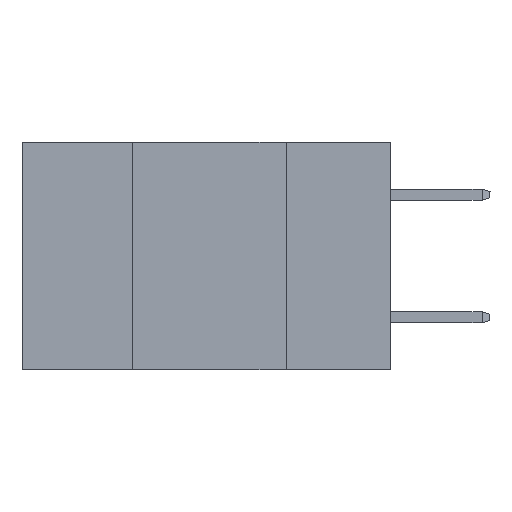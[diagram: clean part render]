
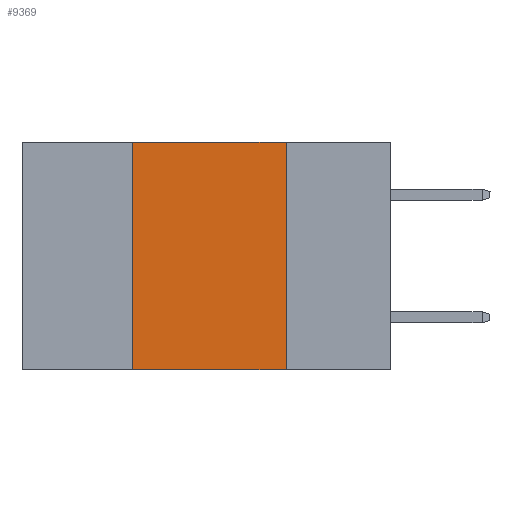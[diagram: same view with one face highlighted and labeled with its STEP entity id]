
A CAD part, left-side view. The second image highlights one B-rep face of the part: STEP entity #9369.
In plain terms, the highlighted planar face has unit normal (-1, 0, 0).
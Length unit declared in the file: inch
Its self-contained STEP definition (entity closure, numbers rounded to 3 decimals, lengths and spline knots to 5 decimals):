
#109 = EDGE_CURVE ( 'NONE', #7183, #10143, #8267, .T. ) ;
#185 = PLANE ( 'NONE',  #5497 ) ;
#631 = DIRECTION ( 'NONE',  ( 0., -1., 0. ) ) ;
#1156 = ORIENTED_EDGE ( 'NONE', *, *, #8294, .F. ) ;
#1459 = VERTEX_POINT ( 'NONE', #3771 ) ;
#1768 = EDGE_LOOP ( 'NONE', ( #2166, #1156, #7335, #7199 ) ) ;
#1783 = CARTESIAN_POINT ( 'NONE',  ( 0., 0.6, 0. ) ) ;
#2166 = ORIENTED_EDGE ( 'NONE', *, *, #109, .F. ) ;
#2233 = CARTESIAN_POINT ( 'NONE',  ( 0., 0.6, 0. ) ) ;
#2931 = VECTOR ( 'NONE', #5662, 39.37008 ) ;
#2969 = VERTEX_POINT ( 'NONE', #10091 ) ;
#3101 = LINE ( 'NONE', #2233, #7583 ) ;
#3521 = DIRECTION ( 'NONE',  ( 0., 0., -1. ) ) ;
#3768 = CARTESIAN_POINT ( 'NONE',  ( 0., 0.17, -0.37 ) ) ;
#3771 = CARTESIAN_POINT ( 'NONE',  ( 0., 0.42, 0. ) ) ;
#4288 = CARTESIAN_POINT ( 'NONE',  ( 0., 0.17, 0. ) ) ;
#5113 = DIRECTION ( 'NONE',  ( 0., -1., 0. ) ) ;
#5120 = VECTOR ( 'NONE', #5113, 39.37008 ) ;
#5497 = AXIS2_PLACEMENT_3D ( 'NONE', #1783, #8742, #8946 ) ;
#5655 = EDGE_CURVE ( 'NONE', #2969, #1459, #6549, .T. ) ;
#5662 = DIRECTION ( 'NONE',  ( 0., 0., 1. ) ) ;
#5839 = LINE ( 'NONE', #9708, #5120 ) ;
#6549 = LINE ( 'NONE', #8803, #2931 ) ;
#7120 = VECTOR ( 'NONE', #3521, 39.37008 ) ;
#7183 = VERTEX_POINT ( 'NONE', #8450 ) ;
#7199 = ORIENTED_EDGE ( 'NONE', *, *, #8623, .T. ) ;
#7335 = ORIENTED_EDGE ( 'NONE', *, *, #5655, .F. ) ;
#7583 = VECTOR ( 'NONE', #631, 39.37008 ) ;
#8132 = FACE_OUTER_BOUND ( 'NONE', #1768, .T. ) ;
#8267 = LINE ( 'NONE', #4288, #7120 ) ;
#8294 = EDGE_CURVE ( 'NONE', #1459, #7183, #3101, .T. ) ;
#8450 = CARTESIAN_POINT ( 'NONE',  ( 0., 0.17, 0. ) ) ;
#8623 = EDGE_CURVE ( 'NONE', #2969, #10143, #5839, .T. ) ;
#8742 = DIRECTION ( 'NONE',  ( 1., 0., 0. ) ) ;
#8803 = CARTESIAN_POINT ( 'NONE',  ( 0., 0.42, 0. ) ) ;
#8946 = DIRECTION ( 'NONE',  ( 0., 0., -1. ) ) ;
#9369 = ADVANCED_FACE ( 'NONE', ( #8132 ), #185, .F. ) ;
#9708 = CARTESIAN_POINT ( 'NONE',  ( 0., 0.6, -0.37 ) ) ;
#10091 = CARTESIAN_POINT ( 'NONE',  ( 0., 0.42, -0.37 ) ) ;
#10143 = VERTEX_POINT ( 'NONE', #3768 ) ;
